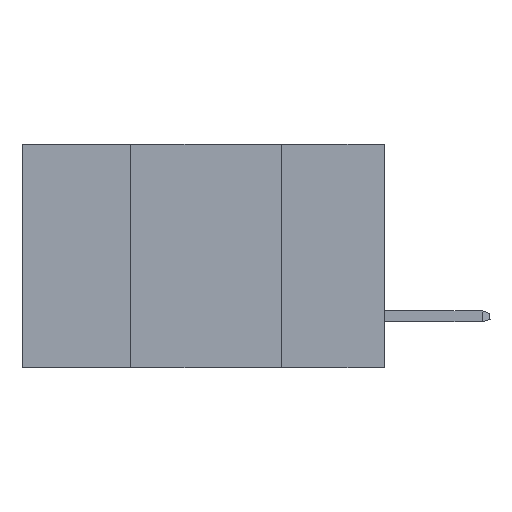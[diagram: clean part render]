
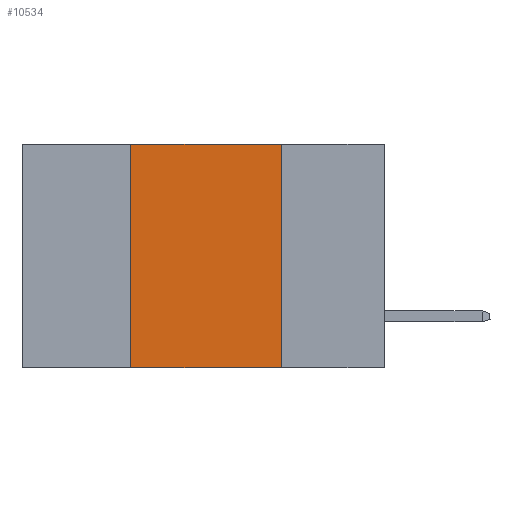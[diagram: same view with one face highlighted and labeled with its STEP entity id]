
A CAD part, left-side view. The second image highlights one B-rep face of the part: STEP entity #10534.
In plain terms, the highlighted planar face has unit normal (-1, 0, 0).
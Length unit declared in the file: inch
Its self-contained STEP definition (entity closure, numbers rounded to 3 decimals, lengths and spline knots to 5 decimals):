
#320 = AXIS2_PLACEMENT_3D ( 'NONE', #6482, #4841, #11482 ) ;
#1201 = EDGE_CURVE ( 'NONE', #21254, #17625, #1358, .T. ) ;
#1358 = LINE ( 'NONE', #5645, #16940 ) ;
#1549 = CARTESIAN_POINT ( 'NONE',  ( 0., 0.42, 0. ) ) ;
#1661 = DIRECTION ( 'NONE',  ( 0., 0., 1. ) ) ;
#2464 = ORIENTED_EDGE ( 'NONE', *, *, #5310, .F. ) ;
#4129 = ORIENTED_EDGE ( 'NONE', *, *, #4627, .T. ) ;
#4175 = DIRECTION ( 'NONE',  ( 0., 0., -1. ) ) ;
#4281 = LINE ( 'NONE', #11340, #9356 ) ;
#4627 = EDGE_CURVE ( 'NONE', #21479, #20495, #18632, .T. ) ;
#4841 = DIRECTION ( 'NONE',  ( 1., 0., 0. ) ) ;
#4845 = LINE ( 'NONE', #11843, #13402 ) ;
#5310 = EDGE_CURVE ( 'NONE', #17625, #20495, #4281, .T. ) ;
#5645 = CARTESIAN_POINT ( 'NONE',  ( 0., 0.6, 0. ) ) ;
#6342 = PLANE ( 'NONE',  #320 ) ;
#6471 = DIRECTION ( 'NONE',  ( 0., -1., 0. ) ) ;
#6482 = CARTESIAN_POINT ( 'NONE',  ( 0., 0.6, 0. ) ) ;
#7409 = ORIENTED_EDGE ( 'NONE', *, *, #18149, .F. ) ;
#9356 = VECTOR ( 'NONE', #4175, 39.37008 ) ;
#10534 = ADVANCED_FACE ( 'NONE', ( #13970 ), #6342, .F. ) ;
#10617 = CARTESIAN_POINT ( 'NONE',  ( 0., 0.17, 0. ) ) ;
#11340 = CARTESIAN_POINT ( 'NONE',  ( 0., 0.17, 0. ) ) ;
#11482 = DIRECTION ( 'NONE',  ( 0., 0., -1. ) ) ;
#11843 = CARTESIAN_POINT ( 'NONE',  ( 0., 0.42, 0. ) ) ;
#12018 = ORIENTED_EDGE ( 'NONE', *, *, #1201, .F. ) ;
#12292 = CARTESIAN_POINT ( 'NONE',  ( 0., 0.17, -0.37 ) ) ;
#12939 = CARTESIAN_POINT ( 'NONE',  ( 0., 0.42, -0.37 ) ) ;
#13402 = VECTOR ( 'NONE', #1661, 39.37008 ) ;
#13970 = FACE_OUTER_BOUND ( 'NONE', #16579, .T. ) ;
#15627 = CARTESIAN_POINT ( 'NONE',  ( 0., 0.6, -0.37 ) ) ;
#16579 = EDGE_LOOP ( 'NONE', ( #2464, #12018, #7409, #4129 ) ) ;
#16940 = VECTOR ( 'NONE', #17574, 39.37008 ) ;
#17574 = DIRECTION ( 'NONE',  ( 0., -1., 0. ) ) ;
#17625 = VERTEX_POINT ( 'NONE', #10617 ) ;
#18149 = EDGE_CURVE ( 'NONE', #21479, #21254, #4845, .T. ) ;
#18632 = LINE ( 'NONE', #15627, #19169 ) ;
#19169 = VECTOR ( 'NONE', #6471, 39.37008 ) ;
#20495 = VERTEX_POINT ( 'NONE', #12292 ) ;
#21254 = VERTEX_POINT ( 'NONE', #1549 ) ;
#21479 = VERTEX_POINT ( 'NONE', #12939 ) ;
